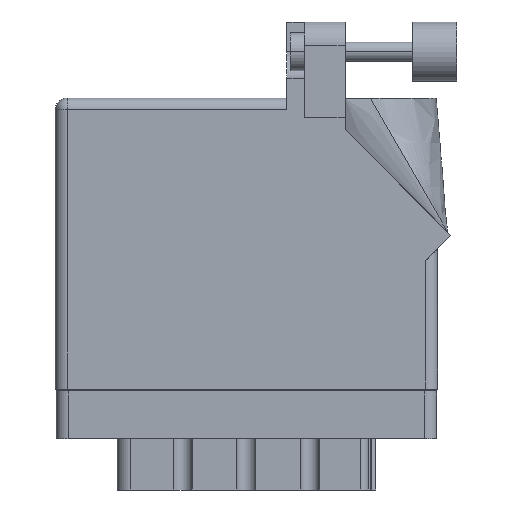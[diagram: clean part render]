
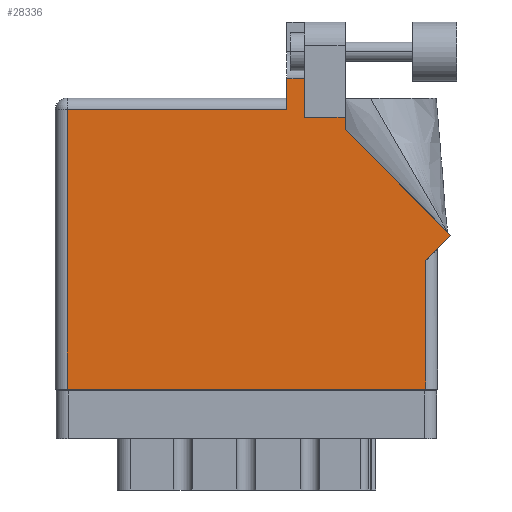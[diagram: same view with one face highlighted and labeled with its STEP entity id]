
A CAD part, front view. The second image highlights one B-rep face of the part: STEP entity #28336.
In plain terms, the highlighted face is planar.
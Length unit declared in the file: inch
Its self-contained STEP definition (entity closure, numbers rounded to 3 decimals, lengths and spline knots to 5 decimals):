
#387 = ORIENTED_EDGE ( 'NONE', *, *, #903, .T. ) ;
#706 = EDGE_CURVE ( 'NONE', #23176, #10110, #20841, .T. ) ;
#814 = CARTESIAN_POINT ( 'NONE',  ( 1.64177, 1.6315, 0. ) ) ;
#903 = EDGE_CURVE ( 'NONE', #10110, #1967, #32399, .T. ) ;
#1040 = LINE ( 'NONE', #3291, #40218 ) ;
#1079 = CARTESIAN_POINT ( 'NONE',  ( 1.524, 1.43, 0. ) ) ;
#1967 = VERTEX_POINT ( 'NONE', #12313 ) ;
#2507 = EDGE_CURVE ( 'NONE', #17740, #35782, #32385, .T. ) ;
#2618 = ORIENTED_EDGE ( 'NONE', *, *, #10181, .T. ) ;
#3004 = ORIENTED_EDGE ( 'NONE', *, *, #37445, .T. ) ;
#3291 = CARTESIAN_POINT ( 'NONE',  ( 1.311, 1.43, 0. ) ) ;
#3363 = VECTOR ( 'NONE', #37939, 39.37008 ) ;
#3718 = VECTOR ( 'NONE', #9452, 39.37008 ) ;
#5202 = VECTOR ( 'NONE', #9009, 39.37008 ) ;
#5234 = LINE ( 'NONE', #6298, #39940 ) ;
#5753 = VECTOR ( 'NONE', #37525, 39.37008 ) ;
#6242 = VECTOR ( 'NONE', #40271, 39.37008 ) ;
#6298 = CARTESIAN_POINT ( 'NONE',  ( 1.524, 1.43, 0. ) ) ;
#8055 = EDGE_CURVE ( 'NONE', #36662, #23176, #1040, .T. ) ;
#9009 = DIRECTION ( 'NONE',  ( 1., 0., 0. ) ) ;
#9175 = DIRECTION ( 'NONE',  ( 0., 1., 0. ) ) ;
#9452 = DIRECTION ( 'NONE',  ( 0., 1., 0. ) ) ;
#10110 = VERTEX_POINT ( 'NONE', #23745 ) ;
#10181 = EDGE_CURVE ( 'NONE', #20278, #16123, #28478, .T. ) ;
#11041 = EDGE_CURVE ( 'NONE', #33816, #36662, #5234, .T. ) ;
#11583 = CARTESIAN_POINT ( 'NONE',  ( 0., 1.53, 0. ) ) ;
#11833 = ORIENTED_EDGE ( 'NONE', *, *, #8055, .T. ) ;
#12134 = CARTESIAN_POINT ( 'NONE',  ( 1.948, 0.737, 0. ) ) ;
#12273 = LINE ( 'NONE', #12134, #3718 ) ;
#12313 = CARTESIAN_POINT ( 'NONE',  ( 1.217, 1.468, 0. ) ) ;
#12929 = EDGE_CURVE ( 'NONE', #20908, #17740, #23442, .T. ) ;
#13709 = DIRECTION ( 'NONE',  ( -1., 0., 0. ) ) ;
#13897 = VERTEX_POINT ( 'NONE', #26760 ) ;
#14059 = ORIENTED_EDGE ( 'NONE', *, *, #35461, .T. ) ;
#14942 = CARTESIAN_POINT ( 'NONE',  ( 1.311, 1.6315, 0. ) ) ;
#15489 = CARTESIAN_POINT ( 'NONE',  ( 0.062, 0., 0. ) ) ;
#16123 = VERTEX_POINT ( 'NONE', #37584 ) ;
#16250 = AXIS2_PLACEMENT_3D ( 'NONE', #11583, #34035, #40758 ) ;
#17740 = VERTEX_POINT ( 'NONE', #24520 ) ;
#18472 = CARTESIAN_POINT ( 'NONE',  ( 1.948, 0.675, 0. ) ) ;
#19486 = CARTESIAN_POINT ( 'NONE',  ( 1.311, 1.43, 0. ) ) ;
#19949 = VECTOR ( 'NONE', #25248, 39.37008 ) ;
#20278 = VERTEX_POINT ( 'NONE', #18472 ) ;
#20841 = LINE ( 'NONE', #814, #37449 ) ;
#20873 = CARTESIAN_POINT ( 'NONE',  ( 0., 1.468, 0. ) ) ;
#20908 = VERTEX_POINT ( 'NONE', #31538 ) ;
#22994 = ORIENTED_EDGE ( 'NONE', *, *, #12929, .T. ) ;
#23176 = VERTEX_POINT ( 'NONE', #14942 ) ;
#23442 = LINE ( 'NONE', #15489, #3363 ) ;
#23653 = VECTOR ( 'NONE', #26906, 39.37008 ) ;
#23745 = CARTESIAN_POINT ( 'NONE',  ( 1.217, 1.6315, 0. ) ) ;
#24520 = CARTESIAN_POINT ( 'NONE',  ( 0.062, 0., 0. ) ) ;
#24636 = CARTESIAN_POINT ( 'NONE',  ( 1.217, 1.53, 0. ) ) ;
#25248 = DIRECTION ( 'NONE',  ( 0.707, 0.707, 0. ) ) ;
#25528 = EDGE_CURVE ( 'NONE', #13897, #33816, #27184, .T. ) ;
#25850 = LINE ( 'NONE', #40131, #6242 ) ;
#26325 = EDGE_LOOP ( 'NONE', ( #11833, #39636, #387, #14059, #22994, #35506, #35918, #2618, #3004, #38045, #34579 ) ) ;
#26760 = CARTESIAN_POINT ( 'NONE',  ( 1.524, 1.36442, 0. ) ) ;
#26906 = DIRECTION ( 'NONE',  ( 0., 1., 0. ) ) ;
#27184 = LINE ( 'NONE', #29837, #23653 ) ;
#28174 = CARTESIAN_POINT ( 'NONE',  ( 2.01, 0.737, 0. ) ) ;
#28336 = ADVANCED_FACE ( 'NONE', ( #37945 ), #40627, .F. ) ;
#28478 = LINE ( 'NONE', #28174, #19949 ) ;
#28783 = DIRECTION ( 'NONE',  ( -1., 0., 0. ) ) ;
#29508 = CARTESIAN_POINT ( 'NONE',  ( 1.948, 0., 0. ) ) ;
#29837 = CARTESIAN_POINT ( 'NONE',  ( 1.524, 1.36442, 0. ) ) ;
#30288 = EDGE_CURVE ( 'NONE', #35782, #20278, #12273, .T. ) ;
#30829 = DIRECTION ( 'NONE',  ( -1., 0., 0. ) ) ;
#31221 = CARTESIAN_POINT ( 'NONE',  ( 0., 0., 0. ) ) ;
#31527 = LINE ( 'NONE', #20873, #41041 ) ;
#31538 = CARTESIAN_POINT ( 'NONE',  ( 0.062, 1.468, 0. ) ) ;
#32385 = LINE ( 'NONE', #31221, #5202 ) ;
#32399 = LINE ( 'NONE', #24636, #5753 ) ;
#33816 = VERTEX_POINT ( 'NONE', #1079 ) ;
#34035 = DIRECTION ( 'NONE',  ( 0., 0., -1. ) ) ;
#34579 = ORIENTED_EDGE ( 'NONE', *, *, #11041, .T. ) ;
#35461 = EDGE_CURVE ( 'NONE', #1967, #20908, #31527, .T. ) ;
#35506 = ORIENTED_EDGE ( 'NONE', *, *, #2507, .T. ) ;
#35782 = VERTEX_POINT ( 'NONE', #29508 ) ;
#35918 = ORIENTED_EDGE ( 'NONE', *, *, #30288, .T. ) ;
#36662 = VERTEX_POINT ( 'NONE', #19486 ) ;
#37445 = EDGE_CURVE ( 'NONE', #16123, #13897, #25850, .T. ) ;
#37449 = VECTOR ( 'NONE', #13709, 39.37008 ) ;
#37525 = DIRECTION ( 'NONE',  ( 0., -1., 0. ) ) ;
#37584 = CARTESIAN_POINT ( 'NONE',  ( 2.08071, 0.80771, 0. ) ) ;
#37939 = DIRECTION ( 'NONE',  ( 0., -1., 0. ) ) ;
#37945 = FACE_OUTER_BOUND ( 'NONE', #26325, .T. ) ;
#38045 = ORIENTED_EDGE ( 'NONE', *, *, #25528, .T. ) ;
#39636 = ORIENTED_EDGE ( 'NONE', *, *, #706, .T. ) ;
#39940 = VECTOR ( 'NONE', #28783, 39.37008 ) ;
#40131 = CARTESIAN_POINT ( 'NONE',  ( 2.08071, 0.80771, 0. ) ) ;
#40218 = VECTOR ( 'NONE', #9175, 39.37008 ) ;
#40271 = DIRECTION ( 'NONE',  ( -0.707, 0.707, 0. ) ) ;
#40627 = PLANE ( 'NONE',  #16250 ) ;
#40758 = DIRECTION ( 'NONE',  ( -1., 0., 0. ) ) ;
#41041 = VECTOR ( 'NONE', #30829, 39.37008 ) ;
